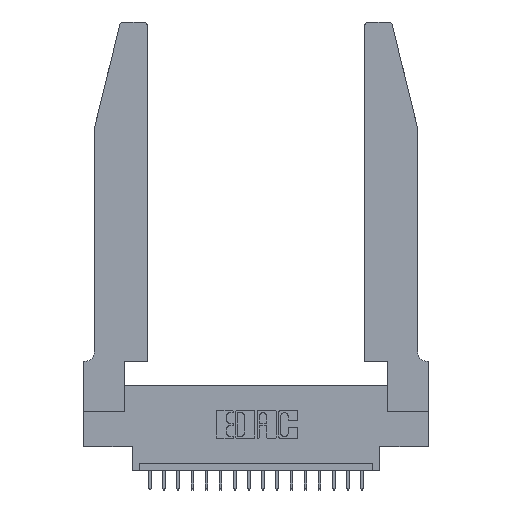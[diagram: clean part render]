
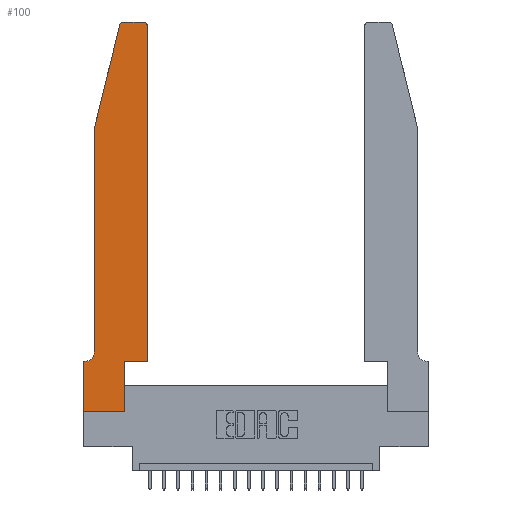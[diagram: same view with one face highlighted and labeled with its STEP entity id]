
A CAD part, top view. The second image highlights one B-rep face of the part: STEP entity #100.
In plain terms, the highlighted planar face has unit normal (0, 0, 1).
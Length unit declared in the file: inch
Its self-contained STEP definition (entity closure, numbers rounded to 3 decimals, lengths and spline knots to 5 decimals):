
#18 = DIRECTION ( 'NONE',  ( -1., 0., 0. ) ) ;
#100 = ADVANCED_FACE ( 'NONE', ( #10176 ), #5694, .T. ) ;
#101 = DIRECTION ( 'NONE',  ( 1., 0., 0. ) ) ;
#285 = VERTEX_POINT ( 'NONE', #2988 ) ;
#385 = ORIENTED_EDGE ( 'NONE', *, *, #2535, .T. ) ;
#459 = CARTESIAN_POINT ( 'NONE',  ( 0.2865, 0.35, 0.37 ) ) ;
#723 = CIRCLE ( 'NONE', #2711, 0.07 ) ;
#930 = DIRECTION ( 'NONE',  ( 1., 0., 0. ) ) ;
#1181 = EDGE_CURVE ( 'NONE', #16364, #10242, #12659, .T. ) ;
#1197 = EDGE_LOOP ( 'NONE', ( #7239, #16066, #15985, #10244, #385, #5467, #17062, #8670, #19810, #9257, #13750, #2581 ) ) ;
#1372 = CARTESIAN_POINT ( 'NONE',  ( 0., 0., 0.37 ) ) ;
#2053 = VECTOR ( 'NONE', #3002, 39.37008 ) ;
#2186 = CARTESIAN_POINT ( 'NONE',  ( 0.25487, 2.72718, 0.37 ) ) ;
#2209 = DIRECTION ( 'NONE',  ( -0.239, -0.971, 0. ) ) ;
#2212 = CIRCLE ( 'NONE', #19407, 0.03 ) ;
#2219 = VECTOR ( 'NONE', #18759, 39.37008 ) ;
#2535 = EDGE_CURVE ( 'NONE', #17929, #9585, #723, .T. ) ;
#2581 = ORIENTED_EDGE ( 'NONE', *, *, #1181, .T. ) ;
#2711 = AXIS2_PLACEMENT_3D ( 'NONE', #13882, #8873, #13976 ) ;
#2988 = CARTESIAN_POINT ( 'NONE',  ( 0.4505, 0.35, 0.37 ) ) ;
#3002 = DIRECTION ( 'NONE',  ( 1., 0., 0. ) ) ;
#3389 = CARTESIAN_POINT ( 'NONE',  ( 0.284, 2.75, 0.37 ) ) ;
#3572 = VECTOR ( 'NONE', #5747, 39.37008 ) ;
#4085 = CARTESIAN_POINT ( 'NONE',  ( 0.4505, 0.35, 0.37 ) ) ;
#4205 = EDGE_CURVE ( 'NONE', #7747, #17929, #13256, .T. ) ;
#4219 = EDGE_CURVE ( 'NONE', #4607, #7747, #19459, .T. ) ;
#4326 = VERTEX_POINT ( 'NONE', #1372 ) ;
#4607 = VERTEX_POINT ( 'NONE', #2186 ) ;
#4638 = AXIS2_PLACEMENT_3D ( 'NONE', #6944, #13414, #930 ) ;
#4700 = VECTOR ( 'NONE', #101, 39.37008 ) ;
#4822 = EDGE_CURVE ( 'NONE', #17138, #285, #12896, .T. ) ;
#4832 = EDGE_CURVE ( 'NONE', #4326, #15665, #7771, .T. ) ;
#5227 = CARTESIAN_POINT ( 'NONE',  ( 0.0755, 2., 0.37 ) ) ;
#5467 = ORIENTED_EDGE ( 'NONE', *, *, #11630, .T. ) ;
#5527 = VERTEX_POINT ( 'NONE', #9876 ) ;
#5694 = PLANE ( 'NONE',  #4638 ) ;
#5747 = DIRECTION ( 'NONE',  ( 0., 1., 0. ) ) ;
#6236 = LINE ( 'NONE', #9670, #14300 ) ;
#6944 = CARTESIAN_POINT ( 'NONE',  ( 0., 0.35, 0.37 ) ) ;
#7209 = LINE ( 'NONE', #4085, #3572 ) ;
#7239 = ORIENTED_EDGE ( 'NONE', *, *, #16385, .T. ) ;
#7326 = AXIS2_PLACEMENT_3D ( 'NONE', #12004, #16674, #15424 ) ;
#7544 = CARTESIAN_POINT ( 'NONE',  ( 0.4505, 2.72, 0.37 ) ) ;
#7747 = VERTEX_POINT ( 'NONE', #9192 ) ;
#7771 = LINE ( 'NONE', #14337, #4700 ) ;
#7916 = EDGE_CURVE ( 'NONE', #15665, #17138, #11262, .T. ) ;
#8137 = CARTESIAN_POINT ( 'NONE',  ( 0.0055, 0.35, 0.37 ) ) ;
#8670 = ORIENTED_EDGE ( 'NONE', *, *, #4832, .T. ) ;
#8873 = DIRECTION ( 'NONE',  ( 0., 0., -1. ) ) ;
#9156 = CARTESIAN_POINT ( 'NONE',  ( 0.4205, 2.75, 0.37 ) ) ;
#9192 = CARTESIAN_POINT ( 'NONE',  ( 0.0755, 2., 0.37 ) ) ;
#9257 = ORIENTED_EDGE ( 'NONE', *, *, #4822, .T. ) ;
#9585 = VERTEX_POINT ( 'NONE', #8137 ) ;
#9670 = CARTESIAN_POINT ( 'NONE',  ( 0.0755, 0.35, 0.37 ) ) ;
#9714 = EDGE_CURVE ( 'NONE', #19643, #4607, #2212, .T. ) ;
#9876 = CARTESIAN_POINT ( 'NONE',  ( 0., 0.35, 0.37 ) ) ;
#10176 = FACE_OUTER_BOUND ( 'NONE', #1197, .T. ) ;
#10242 = VERTEX_POINT ( 'NONE', #9156 ) ;
#10244 = ORIENTED_EDGE ( 'NONE', *, *, #4205, .T. ) ;
#10424 = EDGE_CURVE ( 'NONE', #5527, #4326, #14659, .T. ) ;
#11262 = LINE ( 'NONE', #14800, #16088 ) ;
#11344 = VECTOR ( 'NONE', #2209, 39.37008 ) ;
#11630 = EDGE_CURVE ( 'NONE', #9585, #5527, #6236, .T. ) ;
#12004 = CARTESIAN_POINT ( 'NONE',  ( 0.4205, 2.72, 0.37 ) ) ;
#12019 = VECTOR ( 'NONE', #19755, 39.37008 ) ;
#12442 = LINE ( 'NONE', #18862, #2219 ) ;
#12659 = CIRCLE ( 'NONE', #7326, 0.03 ) ;
#12896 = LINE ( 'NONE', #17237, #2053 ) ;
#13019 = CARTESIAN_POINT ( 'NONE',  ( 0.2865, 0., 0.37 ) ) ;
#13150 = CARTESIAN_POINT ( 'NONE',  ( 0.0755, 2., 0.37 ) ) ;
#13256 = LINE ( 'NONE', #13150, #12019 ) ;
#13414 = DIRECTION ( 'NONE',  ( 0., 0., 1. ) ) ;
#13471 = VECTOR ( 'NONE', #16797, 39.37008 ) ;
#13487 = CARTESIAN_POINT ( 'NONE',  ( 0., 0., 0.37 ) ) ;
#13564 = DIRECTION ( 'NONE',  ( 0., 0., 1. ) ) ;
#13750 = ORIENTED_EDGE ( 'NONE', *, *, #15467, .T. ) ;
#13882 = CARTESIAN_POINT ( 'NONE',  ( 0.0055, 0.42, 0.37 ) ) ;
#13976 = DIRECTION ( 'NONE',  ( -1., 0., 0. ) ) ;
#14300 = VECTOR ( 'NONE', #18, 39.37008 ) ;
#14337 = CARTESIAN_POINT ( 'NONE',  ( 0., 0., 0.37 ) ) ;
#14659 = LINE ( 'NONE', #13487, #13471 ) ;
#14800 = CARTESIAN_POINT ( 'NONE',  ( 0.2865, 0.35, 0.37 ) ) ;
#15424 = DIRECTION ( 'NONE',  ( 1., 0., 0. ) ) ;
#15467 = EDGE_CURVE ( 'NONE', #285, #16364, #7209, .T. ) ;
#15665 = VERTEX_POINT ( 'NONE', #13019 ) ;
#15985 = ORIENTED_EDGE ( 'NONE', *, *, #4219, .T. ) ;
#16066 = ORIENTED_EDGE ( 'NONE', *, *, #9714, .T. ) ;
#16088 = VECTOR ( 'NONE', #19460, 39.37008 ) ;
#16364 = VERTEX_POINT ( 'NONE', #7544 ) ;
#16385 = EDGE_CURVE ( 'NONE', #10242, #19643, #12442, .T. ) ;
#16674 = DIRECTION ( 'NONE',  ( 0., 0., 1. ) ) ;
#16797 = DIRECTION ( 'NONE',  ( 0., -1., 0. ) ) ;
#17062 = ORIENTED_EDGE ( 'NONE', *, *, #10424, .T. ) ;
#17138 = VERTEX_POINT ( 'NONE', #459 ) ;
#17237 = CARTESIAN_POINT ( 'NONE',  ( 0.4505, 0.35, 0.37 ) ) ;
#17911 = CARTESIAN_POINT ( 'NONE',  ( 0.284, 2.72, 0.37 ) ) ;
#17929 = VERTEX_POINT ( 'NONE', #18237 ) ;
#18237 = CARTESIAN_POINT ( 'NONE',  ( 0.0755, 0.42, 0.37 ) ) ;
#18319 = DIRECTION ( 'NONE',  ( 1., 0., 0. ) ) ;
#18759 = DIRECTION ( 'NONE',  ( -1., 0., 0. ) ) ;
#18862 = CARTESIAN_POINT ( 'NONE',  ( 0.2605, 2.75, 0.37 ) ) ;
#19407 = AXIS2_PLACEMENT_3D ( 'NONE', #17911, #13564, #18319 ) ;
#19459 = LINE ( 'NONE', #5227, #11344 ) ;
#19460 = DIRECTION ( 'NONE',  ( 0., 1., 0. ) ) ;
#19643 = VERTEX_POINT ( 'NONE', #3389 ) ;
#19755 = DIRECTION ( 'NONE',  ( 0., -1., 0. ) ) ;
#19810 = ORIENTED_EDGE ( 'NONE', *, *, #7916, .T. ) ;
